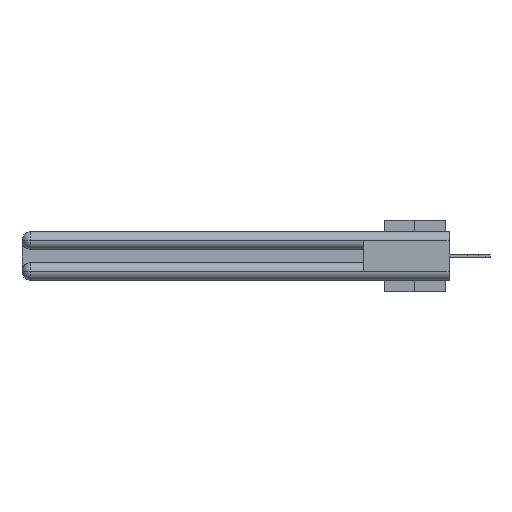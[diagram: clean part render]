
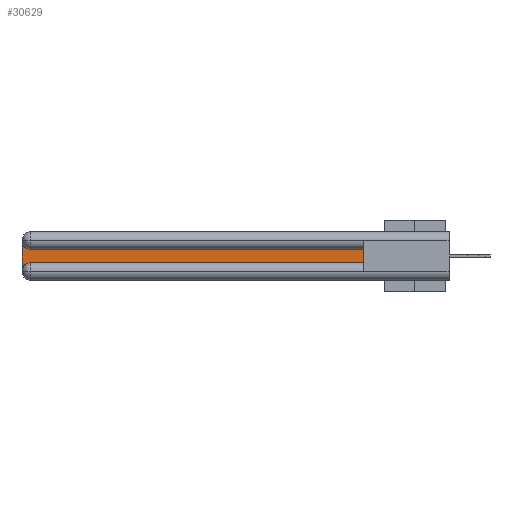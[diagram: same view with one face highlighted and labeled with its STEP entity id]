
A CAD part, left-side view. The second image highlights one B-rep face of the part: STEP entity #30629.
In plain terms, the highlighted planar face has unit normal (-1, 0, 0).
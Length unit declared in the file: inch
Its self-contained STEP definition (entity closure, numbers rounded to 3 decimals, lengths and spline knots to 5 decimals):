
#190 = LINE ( 'NONE', #24209, #19690 ) ;
#598 = CARTESIAN_POINT ( 'NONE',  ( 0.075, 2.94, -0.0625 ) ) ;
#1328 = ORIENTED_EDGE ( 'NONE', *, *, #2732, .T. ) ;
#2635 = EDGE_CURVE ( 'NONE', #22746, #27331, #4680, .T. ) ;
#2717 = DIRECTION ( 'NONE',  ( 1., 0., 0. ) ) ;
#2732 = EDGE_CURVE ( 'NONE', #4710, #22746, #9328, .T. ) ;
#2986 = CARTESIAN_POINT ( 'NONE',  ( 0.075, 0.6, -0.2175 ) ) ;
#4680 = LINE ( 'NONE', #8930, #14404 ) ;
#4710 = VERTEX_POINT ( 'NONE', #23291 ) ;
#4854 = CARTESIAN_POINT ( 'NONE',  ( 0.075, 2.94, -0.2175 ) ) ;
#4903 = EDGE_CURVE ( 'NONE', #27331, #6393, #10344, .T. ) ;
#6373 = VERTEX_POINT ( 'NONE', #31186 ) ;
#6393 = VERTEX_POINT ( 'NONE', #18968 ) ;
#6422 = VERTEX_POINT ( 'NONE', #4854 ) ;
#8930 = CARTESIAN_POINT ( 'NONE',  ( 0.075, 0.6, -0.1225 ) ) ;
#8966 = EDGE_LOOP ( 'NONE', ( #25666, #16280, #17349, #24952, #12861, #1328 ) ) ;
#9328 = LINE ( 'NONE', #2986, #21349 ) ;
#9907 = CARTESIAN_POINT ( 'NONE',  ( 0.075, 3., -0.1225 ) ) ;
#10344 = CIRCLE ( 'NONE', #29687, 0.06 ) ;
#10369 = DIRECTION ( 'NONE',  ( 0., 0., -1. ) ) ;
#10460 = DIRECTION ( 'NONE',  ( 0., 0., 1. ) ) ;
#11519 = EDGE_CURVE ( 'NONE', #6373, #6422, #17860, .T. ) ;
#11681 = DIRECTION ( 'NONE',  ( 0., 0., -1. ) ) ;
#12797 = DIRECTION ( 'NONE',  ( 0., -1., 0. ) ) ;
#12861 = ORIENTED_EDGE ( 'NONE', *, *, #21032, .T. ) ;
#14241 = FACE_OUTER_BOUND ( 'NONE', #8966, .T. ) ;
#14257 = EDGE_CURVE ( 'NONE', #6393, #6373, #190, .T. ) ;
#14404 = VECTOR ( 'NONE', #14637, 39.37008 ) ;
#14637 = DIRECTION ( 'NONE',  ( 0., 1., 0. ) ) ;
#14936 = DIRECTION ( 'NONE',  ( 0., 0., -1. ) ) ;
#16280 = ORIENTED_EDGE ( 'NONE', *, *, #4903, .T. ) ;
#17349 = ORIENTED_EDGE ( 'NONE', *, *, #14257, .T. ) ;
#17812 = CARTESIAN_POINT ( 'NONE',  ( 0.075, 0.6, -0.2175 ) ) ;
#17860 = CIRCLE ( 'NONE', #21243, 0.06 ) ;
#18968 = CARTESIAN_POINT ( 'NONE',  ( 0.075, 3., -0.0625 ) ) ;
#19690 = VECTOR ( 'NONE', #11681, 39.37008 ) ;
#20273 = CARTESIAN_POINT ( 'NONE',  ( 0.075, 2.94, -0.2775 ) ) ;
#20898 = VECTOR ( 'NONE', #12797, 39.37008 ) ;
#21032 = EDGE_CURVE ( 'NONE', #6422, #4710, #26762, .T. ) ;
#21243 = AXIS2_PLACEMENT_3D ( 'NONE', #20273, #22760, #10369 ) ;
#21349 = VECTOR ( 'NONE', #10460, 39.37008 ) ;
#22299 = PLANE ( 'NONE',  #31496 ) ;
#22485 = DIRECTION ( 'NONE',  ( 0., 0., -1. ) ) ;
#22746 = VERTEX_POINT ( 'NONE', #31859 ) ;
#22760 = DIRECTION ( 'NONE',  ( 1., 0., 0. ) ) ;
#23291 = CARTESIAN_POINT ( 'NONE',  ( 0.075, 0.6, -0.2175 ) ) ;
#24209 = CARTESIAN_POINT ( 'NONE',  ( 0.075, 3., -0.2175 ) ) ;
#24952 = ORIENTED_EDGE ( 'NONE', *, *, #11519, .T. ) ;
#25666 = ORIENTED_EDGE ( 'NONE', *, *, #2635, .T. ) ;
#26762 = LINE ( 'NONE', #17812, #20898 ) ;
#27331 = VERTEX_POINT ( 'NONE', #27451 ) ;
#27451 = CARTESIAN_POINT ( 'NONE',  ( 0.075, 2.94, -0.1225 ) ) ;
#27542 = DIRECTION ( 'NONE',  ( 1., 0., 0. ) ) ;
#29687 = AXIS2_PLACEMENT_3D ( 'NONE', #598, #2717, #22485 ) ;
#30629 = ADVANCED_FACE ( 'NONE', ( #14241 ), #22299, .F. ) ;
#31186 = CARTESIAN_POINT ( 'NONE',  ( 0.075, 3., -0.2775 ) ) ;
#31496 = AXIS2_PLACEMENT_3D ( 'NONE', #9907, #27542, #14936 ) ;
#31859 = CARTESIAN_POINT ( 'NONE',  ( 0.075, 0.6, -0.1225 ) ) ;
